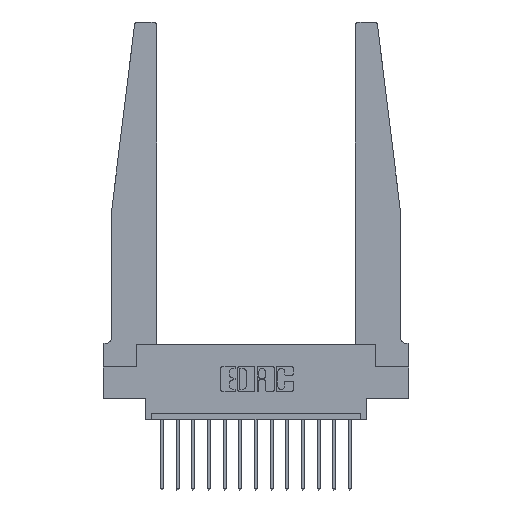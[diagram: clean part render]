
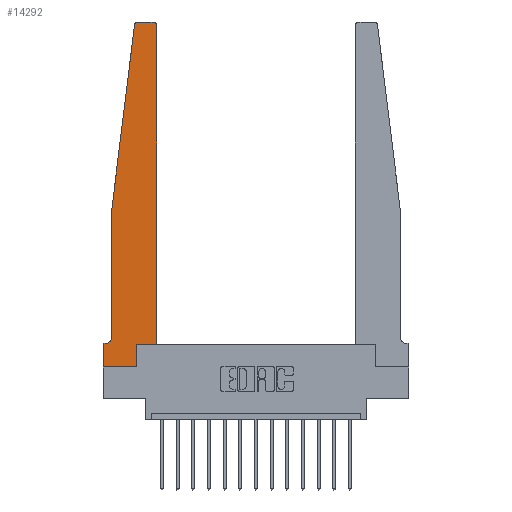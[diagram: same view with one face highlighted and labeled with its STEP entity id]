
A CAD part, top view. The second image highlights one B-rep face of the part: STEP entity #14292.
In plain terms, the highlighted planar face has unit normal (0, 0, 1).
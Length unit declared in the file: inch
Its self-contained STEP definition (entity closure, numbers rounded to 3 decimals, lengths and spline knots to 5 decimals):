
#15 = DIRECTION ( 'NONE',  ( 1., 0., 0. ) ) ;
#107 = VERTEX_POINT ( 'NONE', #719 ) ;
#217 = ORIENTED_EDGE ( 'NONE', *, *, #9212, .T. ) ;
#291 = VERTEX_POINT ( 'NONE', #5092 ) ;
#355 = CARTESIAN_POINT ( 'NONE',  ( 0.425, 2.72, 0.37 ) ) ;
#379 = VECTOR ( 'NONE', #5559, 39.37008 ) ;
#527 = DIRECTION ( 'NONE',  ( 0., 0., -1. ) ) ;
#554 = VERTEX_POINT ( 'NONE', #7812 ) ;
#719 = CARTESIAN_POINT ( 'NONE',  ( 0.2605, 0.18, 0.37 ) ) ;
#1003 = ORIENTED_EDGE ( 'NONE', *, *, #8640, .T. ) ;
#1499 = VECTOR ( 'NONE', #6059, 39.37008 ) ;
#1623 = EDGE_CURVE ( 'NONE', #291, #10335, #12064, .T. ) ;
#1672 = CARTESIAN_POINT ( 'NONE',  ( 0.2605, 0., 0.37 ) ) ;
#1823 = VECTOR ( 'NONE', #15102, 39.37008 ) ;
#1874 = DIRECTION ( 'NONE',  ( 0., 0., 1. ) ) ;
#1953 = LINE ( 'NONE', #4759, #8864 ) ;
#2334 = ORIENTED_EDGE ( 'NONE', *, *, #12781, .T. ) ;
#2401 = VERTEX_POINT ( 'NONE', #15850 ) ;
#2506 = DIRECTION ( 'NONE',  ( 0., 0., 1. ) ) ;
#2607 = VECTOR ( 'NONE', #13831, 39.37008 ) ;
#2649 = VERTEX_POINT ( 'NONE', #3455 ) ;
#2809 = EDGE_CURVE ( 'NONE', #2401, #16917, #9466, .T. ) ;
#2872 = VERTEX_POINT ( 'NONE', #6398 ) ;
#3088 = ORIENTED_EDGE ( 'NONE', *, *, #3835, .T. ) ;
#3128 = CIRCLE ( 'NONE', #16567, 0.05 ) ;
#3275 = DIRECTION ( 'NONE',  ( 0., -1., 0. ) ) ;
#3455 = CARTESIAN_POINT ( 'NONE',  ( 0.065, 1.25, 0.37 ) ) ;
#3469 = CARTESIAN_POINT ( 'NONE',  ( 0., 0.1875, 0.37 ) ) ;
#3503 = ORIENTED_EDGE ( 'NONE', *, *, #8581, .T. ) ;
#3708 = ORIENTED_EDGE ( 'NONE', *, *, #10995, .T. ) ;
#3823 = DIRECTION ( 'NONE',  ( 1., 0., 0. ) ) ;
#3835 = EDGE_CURVE ( 'NONE', #2649, #12338, #4370, .T. ) ;
#4027 = DIRECTION ( 'NONE',  ( -1., 0., 0. ) ) ;
#4370 = LINE ( 'NONE', #9736, #11554 ) ;
#4617 = EDGE_CURVE ( 'NONE', #107, #10142, #9774, .T. ) ;
#4759 = CARTESIAN_POINT ( 'NONE',  ( 0.065, 1.25, 0.37 ) ) ;
#5092 = CARTESIAN_POINT ( 'NONE',  ( 0., 0., 0.37 ) ) ;
#5122 = EDGE_CURVE ( 'NONE', #12338, #2872, #3128, .T. ) ;
#5559 = DIRECTION ( 'NONE',  ( 0., 1., 0. ) ) ;
#5917 = LINE ( 'NONE', #13751, #9203 ) ;
#6007 = AXIS2_PLACEMENT_3D ( 'NONE', #12441, #1874, #16434 ) ;
#6059 = DIRECTION ( 'NONE',  ( 0., 1., 0. ) ) ;
#6107 = ORIENTED_EDGE ( 'NONE', *, *, #2809, .T. ) ;
#6153 = LINE ( 'NONE', #7481, #1499 ) ;
#6226 = CARTESIAN_POINT ( 'NONE',  ( 0.395, 2.75, 0.37 ) ) ;
#6380 = DIRECTION ( 'NONE',  ( 0., 0., 1. ) ) ;
#6398 = CARTESIAN_POINT ( 'NONE',  ( 0.015, 0.1875, 0.37 ) ) ;
#6943 = CARTESIAN_POINT ( 'NONE',  ( 0., 0., 0.37 ) ) ;
#6971 = LINE ( 'NONE', #12347, #2607 ) ;
#7481 = CARTESIAN_POINT ( 'NONE',  ( 0.2605, 0.18, 0.37 ) ) ;
#7812 = CARTESIAN_POINT ( 'NONE',  ( 0., 0.1875, 0.37 ) ) ;
#8097 = CARTESIAN_POINT ( 'NONE',  ( 0.065, 0.1875, 0.37 ) ) ;
#8267 = CIRCLE ( 'NONE', #6007, 0.03 ) ;
#8581 = EDGE_CURVE ( 'NONE', #15215, #2401, #6971, .T. ) ;
#8640 = EDGE_CURVE ( 'NONE', #10142, #14896, #15059, .T. ) ;
#8735 = ORIENTED_EDGE ( 'NONE', *, *, #1623, .T. ) ;
#8864 = VECTOR ( 'NONE', #13911, 39.37008 ) ;
#9203 = VECTOR ( 'NONE', #3275, 39.37008 ) ;
#9212 = EDGE_CURVE ( 'NONE', #10335, #107, #6153, .T. ) ;
#9466 = CIRCLE ( 'NONE', #15348, 0.03 ) ;
#9736 = CARTESIAN_POINT ( 'NONE',  ( 0.065, 1.25, 0.37 ) ) ;
#9774 = LINE ( 'NONE', #16178, #16287 ) ;
#9907 = DIRECTION ( 'NONE',  ( 0., -1., 0. ) ) ;
#9939 = EDGE_CURVE ( 'NONE', #14896, #15215, #8267, .T. ) ;
#10120 = ORIENTED_EDGE ( 'NONE', *, *, #5122, .T. ) ;
#10142 = VERTEX_POINT ( 'NONE', #17026 ) ;
#10243 = VECTOR ( 'NONE', #15, 39.37008 ) ;
#10335 = VERTEX_POINT ( 'NONE', #1672 ) ;
#10440 = CARTESIAN_POINT ( 'NONE',  ( 0.27653, 2.72, 0.37 ) ) ;
#10515 = CARTESIAN_POINT ( 'NONE',  ( 0.065, 0.2375, 0.37 ) ) ;
#10995 = EDGE_CURVE ( 'NONE', #16917, #2649, #1953, .T. ) ;
#11145 = AXIS2_PLACEMENT_3D ( 'NONE', #3469, #6380, #15500 ) ;
#11220 = ORIENTED_EDGE ( 'NONE', *, *, #9939, .T. ) ;
#11554 = VECTOR ( 'NONE', #9907, 39.37008 ) ;
#11849 = PLANE ( 'NONE',  #11145 ) ;
#12064 = LINE ( 'NONE', #6943, #10243 ) ;
#12338 = VERTEX_POINT ( 'NONE', #10515 ) ;
#12347 = CARTESIAN_POINT ( 'NONE',  ( 0.25, 2.75, 0.37 ) ) ;
#12441 = CARTESIAN_POINT ( 'NONE',  ( 0.395, 2.72, 0.37 ) ) ;
#12781 = EDGE_CURVE ( 'NONE', #2872, #554, #16147, .T. ) ;
#13751 = CARTESIAN_POINT ( 'NONE',  ( 0., 0., 0.37 ) ) ;
#13831 = DIRECTION ( 'NONE',  ( -1., 0., 0. ) ) ;
#13911 = DIRECTION ( 'NONE',  ( -0.122, -0.992, 0. ) ) ;
#14234 = EDGE_LOOP ( 'NONE', ( #3503, #6107, #3708, #3088, #10120, #2334, #15156, #8735, #217, #14518, #1003, #11220 ) ) ;
#14280 = CARTESIAN_POINT ( 'NONE',  ( 0.24675, 2.72367, 0.37 ) ) ;
#14292 = ADVANCED_FACE ( 'NONE', ( #14361 ), #11849, .T. ) ;
#14361 = FACE_OUTER_BOUND ( 'NONE', #14234, .T. ) ;
#14518 = ORIENTED_EDGE ( 'NONE', *, *, #4617, .T. ) ;
#14896 = VERTEX_POINT ( 'NONE', #355 ) ;
#14975 = DIRECTION ( 'NONE',  ( 1., 0., 0. ) ) ;
#15059 = LINE ( 'NONE', #15128, #379 ) ;
#15102 = DIRECTION ( 'NONE',  ( -1., 0., 0. ) ) ;
#15128 = CARTESIAN_POINT ( 'NONE',  ( 0.425, 0.18, 0.37 ) ) ;
#15156 = ORIENTED_EDGE ( 'NONE', *, *, #16037, .T. ) ;
#15215 = VERTEX_POINT ( 'NONE', #6226 ) ;
#15348 = AXIS2_PLACEMENT_3D ( 'NONE', #10440, #2506, #3823 ) ;
#15500 = DIRECTION ( 'NONE',  ( 1., 0., 0. ) ) ;
#15850 = CARTESIAN_POINT ( 'NONE',  ( 0.27653, 2.75, 0.37 ) ) ;
#16037 = EDGE_CURVE ( 'NONE', #554, #291, #5917, .T. ) ;
#16067 = CARTESIAN_POINT ( 'NONE',  ( 0.015, 0.2375, 0.37 ) ) ;
#16147 = LINE ( 'NONE', #8097, #1823 ) ;
#16178 = CARTESIAN_POINT ( 'NONE',  ( 0.425, 0.18, 0.37 ) ) ;
#16287 = VECTOR ( 'NONE', #14975, 39.37008 ) ;
#16434 = DIRECTION ( 'NONE',  ( 1., 0., 0. ) ) ;
#16567 = AXIS2_PLACEMENT_3D ( 'NONE', #16067, #527, #4027 ) ;
#16917 = VERTEX_POINT ( 'NONE', #14280 ) ;
#17026 = CARTESIAN_POINT ( 'NONE',  ( 0.425, 0.18, 0.37 ) ) ;
